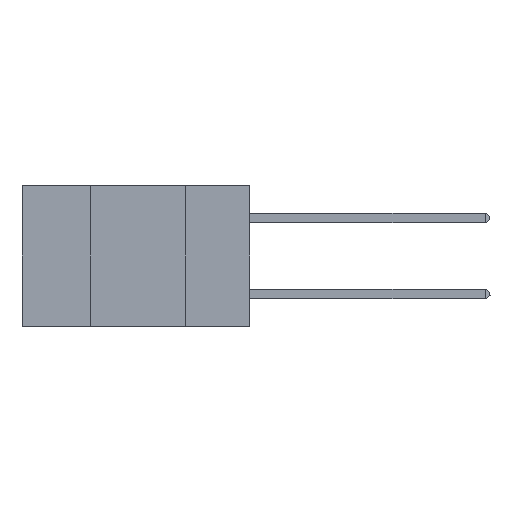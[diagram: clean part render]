
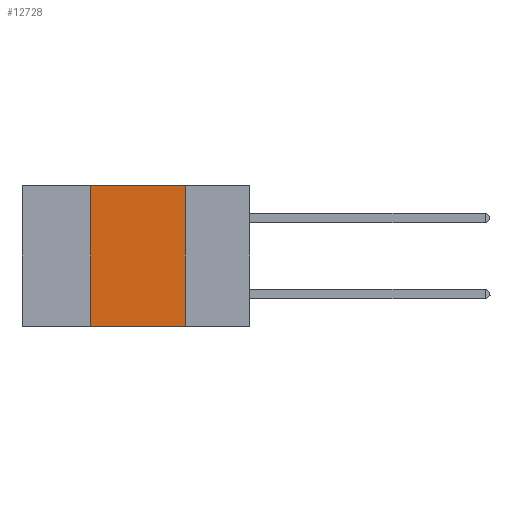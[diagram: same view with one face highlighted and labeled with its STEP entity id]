
A CAD part, left-side view. The second image highlights one B-rep face of the part: STEP entity #12728.
In plain terms, the highlighted planar face has unit normal (-1, 0, 0).
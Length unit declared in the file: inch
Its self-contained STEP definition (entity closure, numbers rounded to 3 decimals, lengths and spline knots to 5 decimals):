
#671 = EDGE_CURVE ( 'NONE', #11746, #10287, #4479, .T. ) ;
#1610 = VECTOR ( 'NONE', #19095, 39.37008 ) ;
#1684 = ORIENTED_EDGE ( 'NONE', *, *, #671, .F. ) ;
#2465 = DIRECTION ( 'NONE',  ( 0., -1., 0. ) ) ;
#3035 = VERTEX_POINT ( 'NONE', #17271 ) ;
#3077 = ORIENTED_EDGE ( 'NONE', *, *, #15451, .F. ) ;
#3609 = CARTESIAN_POINT ( 'NONE',  ( 0., 0.6, 0. ) ) ;
#3848 = EDGE_LOOP ( 'NONE', ( #1684, #3077, #9816, #20015 ) ) ;
#3956 = CARTESIAN_POINT ( 'NONE',  ( 0., 0.6, 0. ) ) ;
#4479 = LINE ( 'NONE', #14268, #22060 ) ;
#5607 = DIRECTION ( 'NONE',  ( 0., 0., -1. ) ) ;
#6980 = LINE ( 'NONE', #3956, #1610 ) ;
#7037 = CARTESIAN_POINT ( 'NONE',  ( 0., 0.17, -0.37 ) ) ;
#8736 = CARTESIAN_POINT ( 'NONE',  ( 0., 0.42, 0. ) ) ;
#9270 = LINE ( 'NONE', #19685, #24497 ) ;
#9776 = FACE_OUTER_BOUND ( 'NONE', #3848, .T. ) ;
#9816 = ORIENTED_EDGE ( 'NONE', *, *, #18194, .F. ) ;
#10287 = VERTEX_POINT ( 'NONE', #7037 ) ;
#10652 = VECTOR ( 'NONE', #13110, 39.37008 ) ;
#11746 = VERTEX_POINT ( 'NONE', #14957 ) ;
#11759 = CARTESIAN_POINT ( 'NONE',  ( 0., 0.42, 0. ) ) ;
#12104 = VERTEX_POINT ( 'NONE', #11759 ) ;
#12156 = DIRECTION ( 'NONE',  ( 0., 0., -1. ) ) ;
#12728 = ADVANCED_FACE ( 'NONE', ( #9776 ), #22964, .F. ) ;
#13110 = DIRECTION ( 'NONE',  ( 0., 0., 1. ) ) ;
#14268 = CARTESIAN_POINT ( 'NONE',  ( 0., 0.17, 0. ) ) ;
#14957 = CARTESIAN_POINT ( 'NONE',  ( 0., 0.17, 0. ) ) ;
#15451 = EDGE_CURVE ( 'NONE', #12104, #11746, #6980, .T. ) ;
#16819 = AXIS2_PLACEMENT_3D ( 'NONE', #3609, #20919, #5607 ) ;
#17271 = CARTESIAN_POINT ( 'NONE',  ( 0., 0.42, -0.37 ) ) ;
#18194 = EDGE_CURVE ( 'NONE', #3035, #12104, #19484, .T. ) ;
#19095 = DIRECTION ( 'NONE',  ( 0., -1., 0. ) ) ;
#19484 = LINE ( 'NONE', #8736, #10652 ) ;
#19685 = CARTESIAN_POINT ( 'NONE',  ( 0., 0.6, -0.37 ) ) ;
#20015 = ORIENTED_EDGE ( 'NONE', *, *, #24539, .T. ) ;
#20919 = DIRECTION ( 'NONE',  ( 1., 0., 0. ) ) ;
#22060 = VECTOR ( 'NONE', #12156, 39.37008 ) ;
#22964 = PLANE ( 'NONE',  #16819 ) ;
#24497 = VECTOR ( 'NONE', #2465, 39.37008 ) ;
#24539 = EDGE_CURVE ( 'NONE', #3035, #10287, #9270, .T. ) ;
